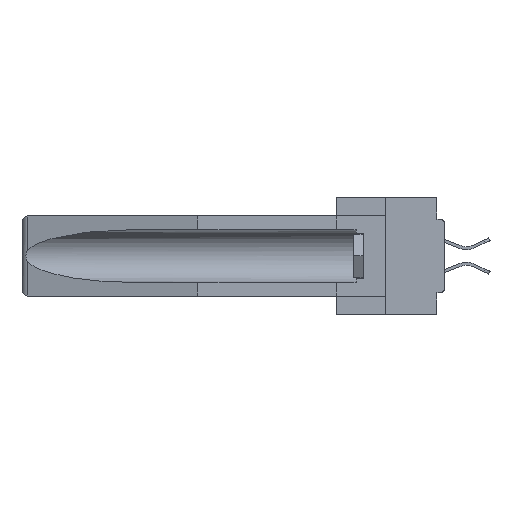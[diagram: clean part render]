
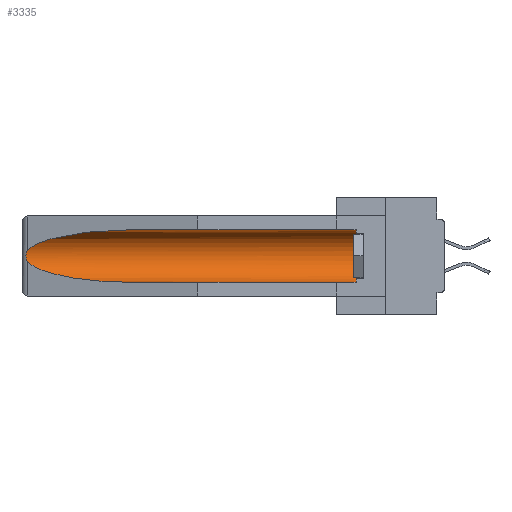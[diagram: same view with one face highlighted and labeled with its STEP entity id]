
A CAD part, left-side view. The second image highlights one B-rep face of the part: STEP entity #3335.
In plain terms, the highlighted cylindrical face has radius 2.857 mm (diameter 5.715 mm), a partial arc.
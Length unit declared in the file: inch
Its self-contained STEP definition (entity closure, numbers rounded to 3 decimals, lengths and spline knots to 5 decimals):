
#505 =( BOUNDED_CURVE ( )  B_SPLINE_CURVE ( 3, ( #7805, #26312, #31709, #15888 ),
 .UNSPECIFIED., .F., .F. ) 
 B_SPLINE_CURVE_WITH_KNOTS ( ( 4, 4 ),
 ( 4.71239, 6.08839 ),
 .UNSPECIFIED. ) 
 CURVE ( )  GEOMETRIC_REPRESENTATION_ITEM ( )  RATIONAL_B_SPLINE_CURVE ( ( 1., 0.848, 0.848, 1. ) ) 
 REPRESENTATION_ITEM ( '' )  );
#829 = CARTESIAN_POINT ( 'NONE',  ( 0.2673, 1.53269, -0.17917 ) ) ;
#861 = FACE_OUTER_BOUND ( 'NONE', #26203, .T. ) ;
#1038 = CARTESIAN_POINT ( 'NONE',  ( 0.26537, 1.52718, -0.14972 ) ) ;
#1156 = CARTESIAN_POINT ( 'NONE',  ( 0.2675, 1.53308, -0.17534 ) ) ;
#1266 = CARTESIAN_POINT ( 'NONE',  ( 0.2673, 1.5327, -0.16383 ) ) ;
#3149 = DIRECTION ( 'NONE',  ( 0., 1., 0. ) ) ;
#3335 = ADVANCED_FACE ( 'NONE', ( #861 ), #30157, .F. ) ;
#4041 = CARTESIAN_POINT ( 'NONE',  ( 0.155, 0.126, -0.1715 ) ) ;
#4643 = EDGE_CURVE ( 'NONE', #9168, #12830, #9947, .T. ) ;
#5278 = ORIENTED_EDGE ( 'NONE', *, *, #7637, .F. ) ;
#6692 =( BOUNDED_CURVE ( )  B_SPLINE_CURVE ( 3, ( #14859, #28470, #22823, #17554 ),
 .UNSPECIFIED., .F., .F. ) 
 B_SPLINE_CURVE_WITH_KNOTS ( ( 4, 4 ),
 ( 0.1948, 1.5708 ),
 .UNSPECIFIED. ) 
 CURVE ( )  GEOMETRIC_REPRESENTATION_ITEM ( )  RATIONAL_B_SPLINE_CURVE ( ( 1., 0.848, 0.848, 1. ) ) 
 REPRESENTATION_ITEM ( '' )  );
#7020 = CARTESIAN_POINT ( 'NONE',  ( 0.155, 1.07973, -0.059 ) ) ;
#7637 = EDGE_CURVE ( 'NONE', #34653, #11444, #8921, .T. ) ;
#7805 = CARTESIAN_POINT ( 'NONE',  ( 0.155, 1.07973, -0.059 ) ) ;
#8921 = LINE ( 'NONE', #10652, #33683 ) ;
#9168 = VERTEX_POINT ( 'NONE', #28248 ) ;
#9947 = LINE ( 'NONE', #14043, #15807 ) ;
#10652 = CARTESIAN_POINT ( 'NONE',  ( 0.155, -0.30754, -0.284 ) ) ;
#11390 = EDGE_CURVE ( 'NONE', #18954, #33816, #16560, .T. ) ;
#11444 = VERTEX_POINT ( 'NONE', #33358 ) ;
#11731 = AXIS2_PLACEMENT_3D ( 'NONE', #4041, #13028, #23209 ) ;
#11884 = CARTESIAN_POINT ( 'NONE',  ( 0.26597, 1.5296, -0.19026 ) ) ;
#12112 = EDGE_CURVE ( 'NONE', #34653, #9168, #27182, .T. ) ;
#12830 = VERTEX_POINT ( 'NONE', #7020 ) ;
#13028 = DIRECTION ( 'NONE',  ( 0., -1., 0. ) ) ;
#14039 = CARTESIAN_POINT ( 'NONE',  ( 0.155, 0.126, -0.284 ) ) ;
#14043 = CARTESIAN_POINT ( 'NONE',  ( 0.155, -0.30754, -0.059 ) ) ;
#14859 = CARTESIAN_POINT ( 'NONE',  ( 0.26537, 1.52718, -0.19328 ) ) ;
#15807 = VECTOR ( 'NONE', #25141, 39.37008 ) ;
#15888 = CARTESIAN_POINT ( 'NONE',  ( 0.26537, 1.52718, -0.14972 ) ) ;
#16560 = B_SPLINE_CURVE_WITH_KNOTS ( 'NONE', 3,
 ( #1038, #17168, #19649, #1266, #27961, #1156, #829, #27514, #11884, #27734 ),
 .UNSPECIFIED., .F., .F.,
 ( 4, 2, 2, 2, 4 ),
 ( 0., 0.00029, 0.00058, 0.00087, 0.00117 ),
 .UNSPECIFIED. ) ;
#16589 = EDGE_CURVE ( 'NONE', #33816, #11444, #6692, .T. ) ;
#17168 = CARTESIAN_POINT ( 'NONE',  ( 0.26597, 1.52961, -0.15275 ) ) ;
#17554 = CARTESIAN_POINT ( 'NONE',  ( 0.155, 1.07973, -0.284 ) ) ;
#18140 = EDGE_CURVE ( 'NONE', #12830, #18954, #505, .T. ) ;
#18954 = VERTEX_POINT ( 'NONE', #28379 ) ;
#19649 = CARTESIAN_POINT ( 'NONE',  ( 0.26654, 1.53092, -0.15636 ) ) ;
#19877 = ORIENTED_EDGE ( 'NONE', *, *, #18140, .T. ) ;
#20671 = ORIENTED_EDGE ( 'NONE', *, *, #16589, .T. ) ;
#22823 = CARTESIAN_POINT ( 'NONE',  ( 0.21114, 1.30732, -0.284 ) ) ;
#23209 = DIRECTION ( 'NONE',  ( 0., 0., 1. ) ) ;
#23654 = CARTESIAN_POINT ( 'NONE',  ( 0.26537, 1.52718, -0.19328 ) ) ;
#25141 = DIRECTION ( 'NONE',  ( 0., 1., 0. ) ) ;
#26203 = EDGE_LOOP ( 'NONE', ( #19877, #28016, #20671, #5278, #30059, #28874 ) ) ;
#26312 = CARTESIAN_POINT ( 'NONE',  ( 0.21114, 1.30732, -0.059 ) ) ;
#27182 = CIRCLE ( 'NONE', #11731, 0.1125 ) ;
#27505 = CARTESIAN_POINT ( 'NONE',  ( 0.155, -0.30754, -0.1715 ) ) ;
#27514 = CARTESIAN_POINT ( 'NONE',  ( 0.26655, 1.53094, -0.18657 ) ) ;
#27734 = CARTESIAN_POINT ( 'NONE',  ( 0.26537, 1.52718, -0.19328 ) ) ;
#27961 = CARTESIAN_POINT ( 'NONE',  ( 0.2675, 1.53308, -0.16763 ) ) ;
#28016 = ORIENTED_EDGE ( 'NONE', *, *, #11390, .T. ) ;
#28248 = CARTESIAN_POINT ( 'NONE',  ( 0.155, 0.126, -0.059 ) ) ;
#28379 = CARTESIAN_POINT ( 'NONE',  ( 0.26537, 1.52718, -0.14972 ) ) ;
#28470 = CARTESIAN_POINT ( 'NONE',  ( 0.25451, 1.48313, -0.24835 ) ) ;
#28874 = ORIENTED_EDGE ( 'NONE', *, *, #4643, .T. ) ;
#30059 = ORIENTED_EDGE ( 'NONE', *, *, #12112, .T. ) ;
#30157 = CYLINDRICAL_SURFACE ( 'NONE', #31058, 0.1125 ) ;
#31058 = AXIS2_PLACEMENT_3D ( 'NONE', #27505, #3149, #33018 ) ;
#31709 = CARTESIAN_POINT ( 'NONE',  ( 0.25451, 1.48313, -0.09465 ) ) ;
#32122 = DIRECTION ( 'NONE',  ( 0., 1., 0. ) ) ;
#33018 = DIRECTION ( 'NONE',  ( 0., 0., 1. ) ) ;
#33358 = CARTESIAN_POINT ( 'NONE',  ( 0.155, 1.07973, -0.284 ) ) ;
#33683 = VECTOR ( 'NONE', #32122, 39.37008 ) ;
#33816 = VERTEX_POINT ( 'NONE', #23654 ) ;
#34653 = VERTEX_POINT ( 'NONE', #14039 ) ;
